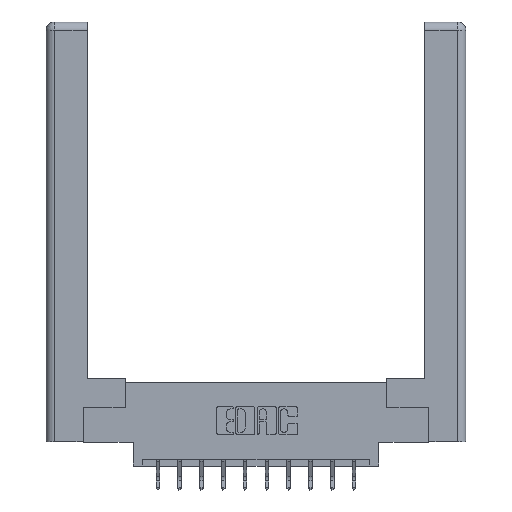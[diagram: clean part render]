
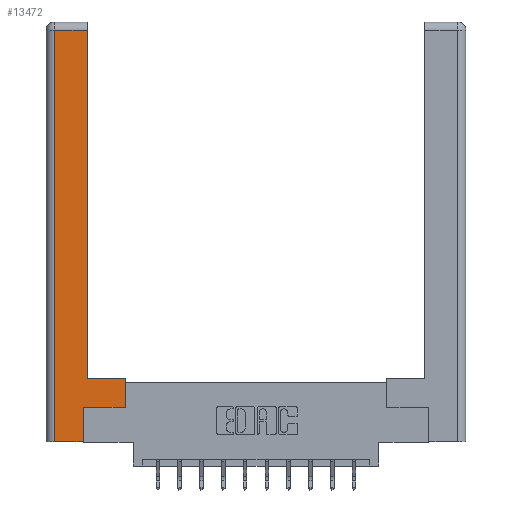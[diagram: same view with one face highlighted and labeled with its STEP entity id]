
A CAD part, top view. The second image highlights one B-rep face of the part: STEP entity #13472.
In plain terms, the highlighted planar face has unit normal (0, 0, 1).
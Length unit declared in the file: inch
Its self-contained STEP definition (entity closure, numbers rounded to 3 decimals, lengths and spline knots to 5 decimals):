
#158 = DIRECTION ( 'NONE',  ( -1., 0., 0. ) ) ;
#258 = CARTESIAN_POINT ( 'NONE',  ( 0., 0., 0. ) ) ;
#263 = LINE ( 'NONE', #4669, #5657 ) ;
#541 = EDGE_CURVE ( 'NONE', #8447, #14570, #11815, .T. ) ;
#753 = EDGE_CURVE ( 'NONE', #2966, #13533, #263, .T. ) ;
#868 = VERTEX_POINT ( 'NONE', #2824 ) ;
#1177 = CARTESIAN_POINT ( 'NONE',  ( 0.565, 0.45, 0. ) ) ;
#1423 = ORIENTED_EDGE ( 'NONE', *, *, #541, .T. ) ;
#1659 = CARTESIAN_POINT ( 'NONE',  ( 0.565, 0.45, 0. ) ) ;
#1710 = DIRECTION ( 'NONE',  ( 0., 1., 0. ) ) ;
#1728 = DIRECTION ( 'NONE',  ( -1., 0., 0. ) ) ;
#2147 = ORIENTED_EDGE ( 'NONE', *, *, #14423, .T. ) ;
#2223 = VECTOR ( 'NONE', #2419, 39.37008 ) ;
#2419 = DIRECTION ( 'NONE',  ( 1., 0., 0. ) ) ;
#2702 = FACE_OUTER_BOUND ( 'NONE', #12576, .T. ) ;
#2824 = CARTESIAN_POINT ( 'NONE',  ( 0.565, 0.245, 0. ) ) ;
#2966 = VERTEX_POINT ( 'NONE', #6839 ) ;
#3063 = CARTESIAN_POINT ( 'NONE',  ( 0.295, 0.45, 0. ) ) ;
#3936 = DIRECTION ( 'NONE',  ( 0., -1., 0. ) ) ;
#4669 = CARTESIAN_POINT ( 'NONE',  ( 0.0615, 2.94, 0. ) ) ;
#4779 = CARTESIAN_POINT ( 'NONE',  ( 0.0615, 2.94, 0. ) ) ;
#5123 = LINE ( 'NONE', #7580, #11984 ) ;
#5136 = VECTOR ( 'NONE', #8203, 39.37008 ) ;
#5412 = ORIENTED_EDGE ( 'NONE', *, *, #14856, .T. ) ;
#5423 = CARTESIAN_POINT ( 'NONE',  ( 0.265, 0., 0. ) ) ;
#5657 = VECTOR ( 'NONE', #158, 39.37008 ) ;
#5770 = LINE ( 'NONE', #5813, #5136 ) ;
#5813 = CARTESIAN_POINT ( 'NONE',  ( 0.295, 3., 0. ) ) ;
#5887 = PLANE ( 'NONE',  #13225 ) ;
#6145 = EDGE_CURVE ( 'NONE', #13533, #6523, #10073, .T. ) ;
#6352 = VECTOR ( 'NONE', #1710, 39.37008 ) ;
#6523 = VERTEX_POINT ( 'NONE', #9437 ) ;
#6839 = CARTESIAN_POINT ( 'NONE',  ( 0.295, 2.94, 0. ) ) ;
#6998 = ORIENTED_EDGE ( 'NONE', *, *, #13973, .T. ) ;
#7337 = ORIENTED_EDGE ( 'NONE', *, *, #753, .T. ) ;
#7580 = CARTESIAN_POINT ( 'NONE',  ( 0.265, 0., 0. ) ) ;
#7716 = VECTOR ( 'NONE', #3936, 39.37008 ) ;
#7994 = LINE ( 'NONE', #9319, #2223 ) ;
#8203 = DIRECTION ( 'NONE',  ( 0., 1., 0. ) ) ;
#8323 = DIRECTION ( 'NONE',  ( 0., 0., -1. ) ) ;
#8420 = ORIENTED_EDGE ( 'NONE', *, *, #6145, .T. ) ;
#8447 = VERTEX_POINT ( 'NONE', #1177 ) ;
#8637 = CARTESIAN_POINT ( 'NONE',  ( 0.295, 0.45, 0. ) ) ;
#8652 = ORIENTED_EDGE ( 'NONE', *, *, #10580, .T. ) ;
#8697 = VERTEX_POINT ( 'NONE', #5423 ) ;
#8720 = LINE ( 'NONE', #1659, #6352 ) ;
#9052 = CARTESIAN_POINT ( 'NONE',  ( 0.265, 0.245, 0. ) ) ;
#9255 = CARTESIAN_POINT ( 'NONE',  ( 0.265, 0.245, 0. ) ) ;
#9295 = LINE ( 'NONE', #9255, #12348 ) ;
#9319 = CARTESIAN_POINT ( 'NONE',  ( 0.565, 0.245, 0. ) ) ;
#9437 = CARTESIAN_POINT ( 'NONE',  ( 0.0615, 0., 0. ) ) ;
#10073 = LINE ( 'NONE', #10864, #7716 ) ;
#10580 = EDGE_CURVE ( 'NONE', #8697, #14180, #9295, .T. ) ;
#10636 = EDGE_CURVE ( 'NONE', #14570, #2966, #5770, .T. ) ;
#10864 = CARTESIAN_POINT ( 'NONE',  ( 0.0615, 0., 0. ) ) ;
#11429 = DIRECTION ( 'NONE',  ( 0., 1., 0. ) ) ;
#11815 = LINE ( 'NONE', #8637, #14310 ) ;
#11984 = VECTOR ( 'NONE', #14452, 39.37008 ) ;
#12348 = VECTOR ( 'NONE', #11429, 39.37008 ) ;
#12576 = EDGE_LOOP ( 'NONE', ( #12817, #7337, #8420, #2147, #8652, #6998, #5412, #1423 ) ) ;
#12817 = ORIENTED_EDGE ( 'NONE', *, *, #10636, .T. ) ;
#13225 = AXIS2_PLACEMENT_3D ( 'NONE', #258, #8323, #13958 ) ;
#13472 = ADVANCED_FACE ( 'NONE', ( #2702 ), #5887, .F. ) ;
#13533 = VERTEX_POINT ( 'NONE', #4779 ) ;
#13958 = DIRECTION ( 'NONE',  ( -1., 0., 0. ) ) ;
#13973 = EDGE_CURVE ( 'NONE', #14180, #868, #7994, .T. ) ;
#14180 = VERTEX_POINT ( 'NONE', #9052 ) ;
#14310 = VECTOR ( 'NONE', #1728, 39.37008 ) ;
#14423 = EDGE_CURVE ( 'NONE', #6523, #8697, #5123, .T. ) ;
#14452 = DIRECTION ( 'NONE',  ( 1., 0., 0. ) ) ;
#14570 = VERTEX_POINT ( 'NONE', #3063 ) ;
#14856 = EDGE_CURVE ( 'NONE', #868, #8447, #8720, .T. ) ;
